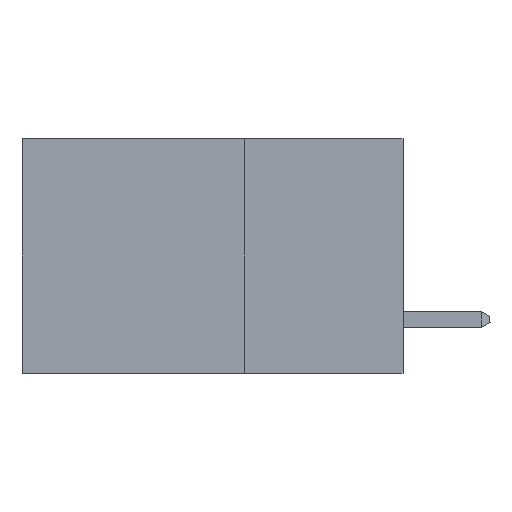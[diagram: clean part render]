
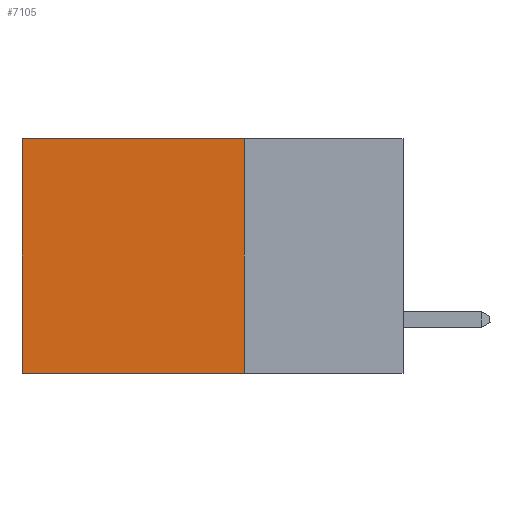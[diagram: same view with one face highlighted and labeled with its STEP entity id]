
A CAD part, left-side view. The second image highlights one B-rep face of the part: STEP entity #7105.
In plain terms, the highlighted planar face has unit normal (-1, 0, 0).
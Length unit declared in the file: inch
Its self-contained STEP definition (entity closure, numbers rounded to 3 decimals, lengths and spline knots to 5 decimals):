
#389 = VERTEX_POINT ( 'NONE', #14999 ) ;
#620 = DIRECTION ( 'NONE',  ( 0., 0., -1. ) ) ;
#815 = LINE ( 'NONE', #20001, #6924 ) ;
#1449 = VECTOR ( 'NONE', #8717, 39.37008 ) ;
#2794 = DIRECTION ( 'NONE',  ( 0., 1., 0. ) ) ;
#2943 = VECTOR ( 'NONE', #620, 39.37008 ) ;
#3300 = EDGE_CURVE ( 'NONE', #389, #15477, #23090, .T. ) ;
#3662 = ORIENTED_EDGE ( 'NONE', *, *, #4929, .F. ) ;
#4253 = CARTESIAN_POINT ( 'NONE',  ( 0.2875, 0.25, -0.37 ) ) ;
#4929 = EDGE_CURVE ( 'NONE', #12529, #15477, #815, .T. ) ;
#5231 = LINE ( 'NONE', #16412, #1449 ) ;
#5356 = FACE_OUTER_BOUND ( 'NONE', #17537, .T. ) ;
#6924 = VECTOR ( 'NONE', #2794, 39.37008 ) ;
#7105 = ADVANCED_FACE ( 'NONE', ( #5356 ), #16005, .F. ) ;
#8406 = CARTESIAN_POINT ( 'NONE',  ( 0.2875, 0.25, 0. ) ) ;
#8717 = DIRECTION ( 'NONE',  ( 0., 1., 0. ) ) ;
#8933 = EDGE_CURVE ( 'NONE', #11595, #12529, #15510, .T. ) ;
#9804 = CARTESIAN_POINT ( 'NONE',  ( 0.2875, 0.25, 0. ) ) ;
#9972 = EDGE_CURVE ( 'NONE', #11595, #389, #5231, .T. ) ;
#10061 = CARTESIAN_POINT ( 'NONE',  ( 0.2875, 0.6, 0. ) ) ;
#11120 = VECTOR ( 'NONE', #21648, 39.37008 ) ;
#11595 = VERTEX_POINT ( 'NONE', #8406 ) ;
#12296 = DIRECTION ( 'NONE',  ( 1., 0., 0. ) ) ;
#12529 = VERTEX_POINT ( 'NONE', #4253 ) ;
#12687 = ORIENTED_EDGE ( 'NONE', *, *, #3300, .T. ) ;
#14999 = CARTESIAN_POINT ( 'NONE',  ( 0.2875, 0.6, 0. ) ) ;
#15477 = VERTEX_POINT ( 'NONE', #18424 ) ;
#15510 = LINE ( 'NONE', #9804, #11120 ) ;
#16005 = PLANE ( 'NONE',  #17520 ) ;
#16373 = ORIENTED_EDGE ( 'NONE', *, *, #9972, .T. ) ;
#16412 = CARTESIAN_POINT ( 'NONE',  ( 0.2875, 0.25, 0. ) ) ;
#17520 = AXIS2_PLACEMENT_3D ( 'NONE', #23715, #12296, #18167 ) ;
#17537 = EDGE_LOOP ( 'NONE', ( #12687, #3662, #18959, #16373 ) ) ;
#18167 = DIRECTION ( 'NONE',  ( 0., 0., -1. ) ) ;
#18424 = CARTESIAN_POINT ( 'NONE',  ( 0.2875, 0.6, -0.37 ) ) ;
#18959 = ORIENTED_EDGE ( 'NONE', *, *, #8933, .F. ) ;
#20001 = CARTESIAN_POINT ( 'NONE',  ( 0.2875, 0.25, -0.37 ) ) ;
#21648 = DIRECTION ( 'NONE',  ( 0., 0., -1. ) ) ;
#23090 = LINE ( 'NONE', #10061, #2943 ) ;
#23715 = CARTESIAN_POINT ( 'NONE',  ( 0.2875, 0.25, 0. ) ) ;
